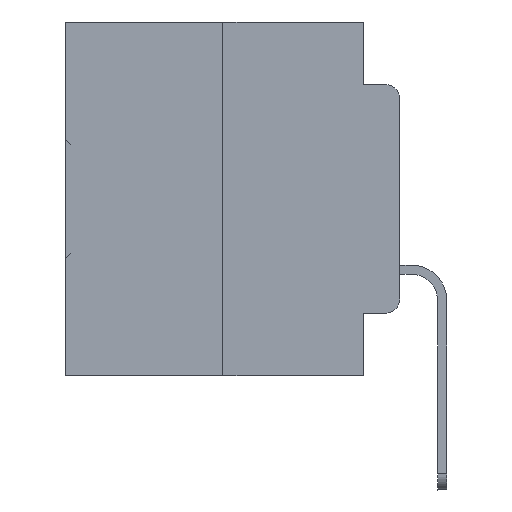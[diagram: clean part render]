
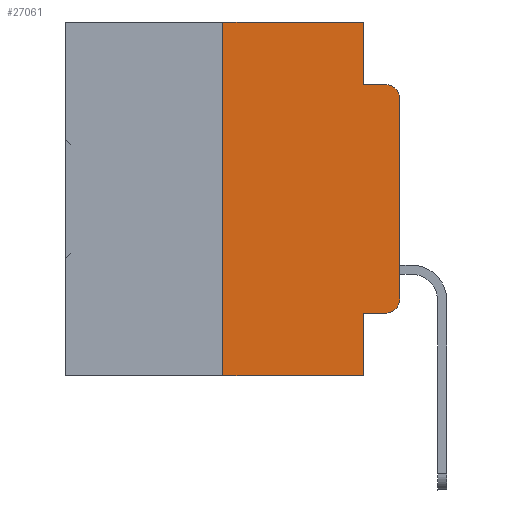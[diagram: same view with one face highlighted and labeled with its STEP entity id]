
A CAD part, left-side view. The second image highlights one B-rep face of the part: STEP entity #27061.
In plain terms, the highlighted planar face has unit normal (-1, 0, 0).
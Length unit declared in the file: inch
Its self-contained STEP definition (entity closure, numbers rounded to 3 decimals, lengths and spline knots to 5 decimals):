
#85 = DIRECTION ( 'NONE',  ( 1., 0., 0. ) ) ;
#264 = VECTOR ( 'NONE', #11286, 39.37008 ) ;
#478 = CARTESIAN_POINT ( 'NONE',  ( 0., 0.051, -0.4115 ) ) ;
#605 = CARTESIAN_POINT ( 'NONE',  ( 0., 0.051, 0. ) ) ;
#945 = LINE ( 'NONE', #26121, #30180 ) ;
#967 = VERTEX_POINT ( 'NONE', #10345 ) ;
#1708 = VECTOR ( 'NONE', #28541, 39.37008 ) ;
#2697 = EDGE_LOOP ( 'NONE', ( #28006, #8385, #6006, #15770, #33647, #23364, #6634, #5149, #15808, #11356 ) ) ;
#3327 = DIRECTION ( 'NONE',  ( 0., 0., -1. ) ) ;
#3829 = DIRECTION ( 'NONE',  ( 0., -1., 0. ) ) ;
#5149 = ORIENTED_EDGE ( 'NONE', *, *, #24170, .F. ) ;
#5328 = EDGE_CURVE ( 'NONE', #12994, #11701, #24461, .T. ) ;
#5937 = CARTESIAN_POINT ( 'NONE',  ( 0., 0.051, -0.5 ) ) ;
#6004 = DIRECTION ( 'NONE',  ( 0., -1., 0. ) ) ;
#6006 = ORIENTED_EDGE ( 'NONE', *, *, #25025, .F. ) ;
#6553 = LINE ( 'NONE', #17261, #26877 ) ;
#6634 = ORIENTED_EDGE ( 'NONE', *, *, #23378, .T. ) ;
#8086 = FACE_OUTER_BOUND ( 'NONE', #2697, .T. ) ;
#8385 = ORIENTED_EDGE ( 'NONE', *, *, #18232, .T. ) ;
#9016 = LINE ( 'NONE', #478, #32251 ) ;
#9152 = DIRECTION ( 'NONE',  ( 0., 0., -1. ) ) ;
#9256 = EDGE_CURVE ( 'NONE', #19490, #33268, #945, .T. ) ;
#10086 = DIRECTION ( 'NONE',  ( 0., 0., -1. ) ) ;
#10345 = CARTESIAN_POINT ( 'NONE',  ( 0., 0.25, -0.5 ) ) ;
#11286 = DIRECTION ( 'NONE',  ( 0., 0., 1. ) ) ;
#11356 = ORIENTED_EDGE ( 'NONE', *, *, #34209, .T. ) ;
#11624 = CARTESIAN_POINT ( 'NONE',  ( 0., 0.051, -0.0885 ) ) ;
#11701 = VERTEX_POINT ( 'NONE', #21128 ) ;
#11936 = CARTESIAN_POINT ( 'NONE',  ( 0., 0.051, -0.0885 ) ) ;
#11979 = LINE ( 'NONE', #11624, #26615 ) ;
#12701 = CARTESIAN_POINT ( 'NONE',  ( 0., 0.051, -0.4115 ) ) ;
#12994 = VERTEX_POINT ( 'NONE', #18941 ) ;
#13415 = AXIS2_PLACEMENT_3D ( 'NONE', #34368, #34903, #10086 ) ;
#13529 = VECTOR ( 'NONE', #24814, 39.37008 ) ;
#14401 = DIRECTION ( 'NONE',  ( -1., 0., 0. ) ) ;
#14907 = VERTEX_POINT ( 'NONE', #12701 ) ;
#15641 = CARTESIAN_POINT ( 'NONE',  ( 0., 0.02, -0.4115 ) ) ;
#15770 = ORIENTED_EDGE ( 'NONE', *, *, #9256, .F. ) ;
#15808 = ORIENTED_EDGE ( 'NONE', *, *, #26785, .T. ) ;
#15935 = EDGE_CURVE ( 'NONE', #967, #28242, #35738, .T. ) ;
#15986 = EDGE_CURVE ( 'NONE', #28242, #19490, #6553, .T. ) ;
#17261 = CARTESIAN_POINT ( 'NONE',  ( 0., 0.473, 0. ) ) ;
#18232 = EDGE_CURVE ( 'NONE', #11701, #31608, #18301, .T. ) ;
#18301 = CIRCLE ( 'NONE', #24626, 0.02 ) ;
#18941 = CARTESIAN_POINT ( 'NONE',  ( 0., 0., -0.3915 ) ) ;
#19153 = PLANE ( 'NONE',  #25219 ) ;
#19490 = VERTEX_POINT ( 'NONE', #605 ) ;
#21128 = CARTESIAN_POINT ( 'NONE',  ( 0., 0., -0.1085 ) ) ;
#21928 = VECTOR ( 'NONE', #22891, 39.37008 ) ;
#22891 = DIRECTION ( 'NONE',  ( 0., -1., 0. ) ) ;
#23060 = DIRECTION ( 'NONE',  ( 0., 0., -1. ) ) ;
#23249 = CARTESIAN_POINT ( 'NONE',  ( 0., 0.473, -0.5 ) ) ;
#23364 = ORIENTED_EDGE ( 'NONE', *, *, #15935, .F. ) ;
#23378 = EDGE_CURVE ( 'NONE', #967, #35641, #28493, .T. ) ;
#23680 = CARTESIAN_POINT ( 'NONE',  ( 0., 0.25, 0. ) ) ;
#24170 = EDGE_CURVE ( 'NONE', #14907, #35641, #31452, .T. ) ;
#24461 = LINE ( 'NONE', #32984, #13529 ) ;
#24626 = AXIS2_PLACEMENT_3D ( 'NONE', #24886, #14401, #3327 ) ;
#24814 = DIRECTION ( 'NONE',  ( 0., 0., 1. ) ) ;
#24886 = CARTESIAN_POINT ( 'NONE',  ( 0., 0.02, -0.1085 ) ) ;
#24913 = CARTESIAN_POINT ( 'NONE',  ( 0., 0.473, 0. ) ) ;
#25025 = EDGE_CURVE ( 'NONE', #33268, #31608, #11979, .T. ) ;
#25219 = AXIS2_PLACEMENT_3D ( 'NONE', #24913, #85, #9152 ) ;
#26121 = CARTESIAN_POINT ( 'NONE',  ( 0., 0.051, 0. ) ) ;
#26615 = VECTOR ( 'NONE', #6004, 39.37008 ) ;
#26785 = EDGE_CURVE ( 'NONE', #14907, #29097, #9016, .T. ) ;
#26877 = VECTOR ( 'NONE', #3829, 39.37008 ) ;
#27061 = ADVANCED_FACE ( 'NONE', ( #8086 ), #19153, .F. ) ;
#27855 = CIRCLE ( 'NONE', #13415, 0.02 ) ;
#28006 = ORIENTED_EDGE ( 'NONE', *, *, #5328, .T. ) ;
#28242 = VERTEX_POINT ( 'NONE', #23680 ) ;
#28493 = LINE ( 'NONE', #23249, #21928 ) ;
#28541 = DIRECTION ( 'NONE',  ( 0., 0., -1. ) ) ;
#29097 = VERTEX_POINT ( 'NONE', #15641 ) ;
#30180 = VECTOR ( 'NONE', #23060, 39.37008 ) ;
#30793 = CARTESIAN_POINT ( 'NONE',  ( 0., 0.02, -0.0885 ) ) ;
#31452 = LINE ( 'NONE', #33995, #1708 ) ;
#31608 = VERTEX_POINT ( 'NONE', #30793 ) ;
#32251 = VECTOR ( 'NONE', #34198, 39.37008 ) ;
#32984 = CARTESIAN_POINT ( 'NONE',  ( 0., 0., 0. ) ) ;
#33016 = CARTESIAN_POINT ( 'NONE',  ( 0., 0.25, 0. ) ) ;
#33268 = VERTEX_POINT ( 'NONE', #11936 ) ;
#33647 = ORIENTED_EDGE ( 'NONE', *, *, #15986, .F. ) ;
#33995 = CARTESIAN_POINT ( 'NONE',  ( 0., 0.051, 0. ) ) ;
#34198 = DIRECTION ( 'NONE',  ( 0., -1., 0. ) ) ;
#34209 = EDGE_CURVE ( 'NONE', #29097, #12994, #27855, .T. ) ;
#34368 = CARTESIAN_POINT ( 'NONE',  ( 0., 0.02, -0.3915 ) ) ;
#34903 = DIRECTION ( 'NONE',  ( -1., 0., 0. ) ) ;
#35641 = VERTEX_POINT ( 'NONE', #5937 ) ;
#35738 = LINE ( 'NONE', #33016, #264 ) ;
